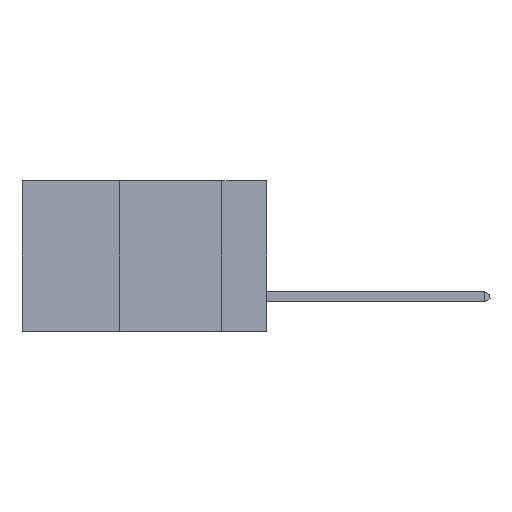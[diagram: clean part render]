
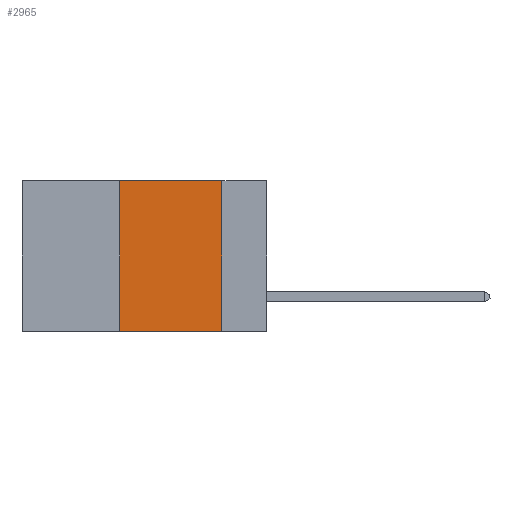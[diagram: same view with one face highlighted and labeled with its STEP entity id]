
A CAD part, left-side view. The second image highlights one B-rep face of the part: STEP entity #2965.
In plain terms, the highlighted planar face has unit normal (-1, 0, 0).
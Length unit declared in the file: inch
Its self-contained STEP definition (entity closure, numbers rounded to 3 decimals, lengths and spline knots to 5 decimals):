
#212 = ORIENTED_EDGE ( 'NONE', *, *, #2498, .F. ) ;
#1181 = CARTESIAN_POINT ( 'NONE',  ( 0., 0.11, 0. ) ) ;
#1563 = LINE ( 'NONE', #3460, #11571 ) ;
#1673 = CARTESIAN_POINT ( 'NONE',  ( 0., 0.6, 0. ) ) ;
#2403 = CARTESIAN_POINT ( 'NONE',  ( 0., 0.6, 0. ) ) ;
#2443 = PLANE ( 'NONE',  #7372 ) ;
#2498 = EDGE_CURVE ( 'NONE', #5715, #6533, #4723, .T. ) ;
#2681 = VECTOR ( 'NONE', #3505, 39.37008 ) ;
#2965 = ADVANCED_FACE ( 'NONE', ( #5909 ), #2443, .F. ) ;
#3105 = CARTESIAN_POINT ( 'NONE',  ( 0., 0.36, 0. ) ) ;
#3303 = DIRECTION ( 'NONE',  ( 1., 0., 0. ) ) ;
#3460 = CARTESIAN_POINT ( 'NONE',  ( 0., 0.36, 0. ) ) ;
#3505 = DIRECTION ( 'NONE',  ( 0., -1., 0. ) ) ;
#4723 = LINE ( 'NONE', #1673, #2681 ) ;
#5154 = EDGE_CURVE ( 'NONE', #9751, #7723, #11914, .T. ) ;
#5715 = VERTEX_POINT ( 'NONE', #3105 ) ;
#5725 = ORIENTED_EDGE ( 'NONE', *, *, #9810, .F. ) ;
#5895 = DIRECTION ( 'NONE',  ( 0., 0., -1. ) ) ;
#5909 = FACE_OUTER_BOUND ( 'NONE', #7041, .T. ) ;
#5927 = CARTESIAN_POINT ( 'NONE',  ( 0., 0.11, 0. ) ) ;
#6184 = VECTOR ( 'NONE', #5895, 39.37008 ) ;
#6533 = VERTEX_POINT ( 'NONE', #1181 ) ;
#7011 = VECTOR ( 'NONE', #10587, 39.37008 ) ;
#7041 = EDGE_LOOP ( 'NONE', ( #5725, #212, #8711, #11179 ) ) ;
#7140 = DIRECTION ( 'NONE',  ( 0., 0., 1. ) ) ;
#7372 = AXIS2_PLACEMENT_3D ( 'NONE', #2403, #3303, #9795 ) ;
#7723 = VERTEX_POINT ( 'NONE', #8029 ) ;
#8029 = CARTESIAN_POINT ( 'NONE',  ( 0., 0.11, -0.37 ) ) ;
#8711 = ORIENTED_EDGE ( 'NONE', *, *, #9133, .F. ) ;
#8728 = CARTESIAN_POINT ( 'NONE',  ( 0., 0.6, -0.37 ) ) ;
#8805 = LINE ( 'NONE', #5927, #6184 ) ;
#9133 = EDGE_CURVE ( 'NONE', #9751, #5715, #1563, .T. ) ;
#9180 = CARTESIAN_POINT ( 'NONE',  ( 0., 0.36, -0.37 ) ) ;
#9751 = VERTEX_POINT ( 'NONE', #9180 ) ;
#9795 = DIRECTION ( 'NONE',  ( 0., 0., -1. ) ) ;
#9810 = EDGE_CURVE ( 'NONE', #6533, #7723, #8805, .T. ) ;
#10587 = DIRECTION ( 'NONE',  ( 0., -1., 0. ) ) ;
#11179 = ORIENTED_EDGE ( 'NONE', *, *, #5154, .T. ) ;
#11571 = VECTOR ( 'NONE', #7140, 39.37008 ) ;
#11914 = LINE ( 'NONE', #8728, #7011 ) ;
